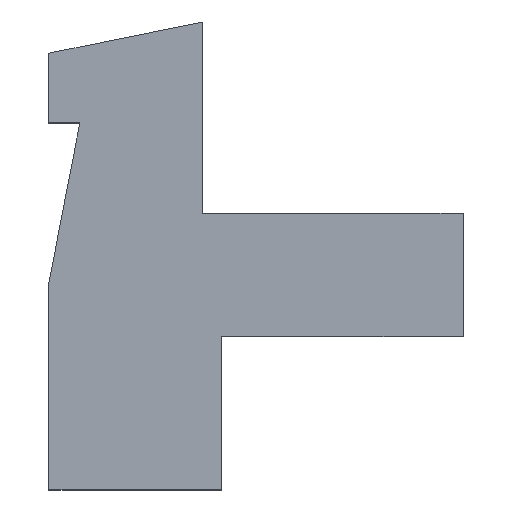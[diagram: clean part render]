
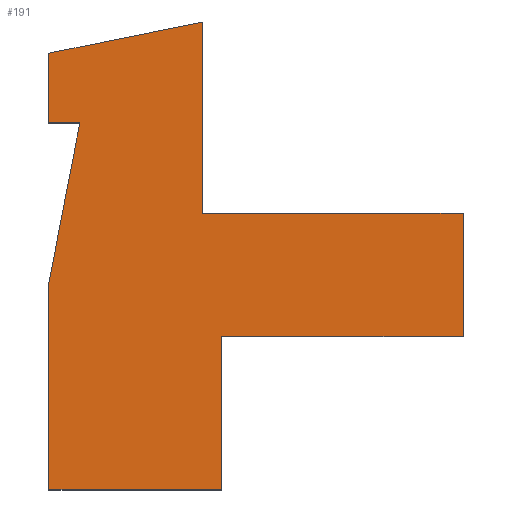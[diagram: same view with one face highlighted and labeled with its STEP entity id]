
A CAD part, top view. The second image highlights one B-rep face of the part: STEP entity #191.
In plain terms, the highlighted planar face has unit normal (0, 0, 1).
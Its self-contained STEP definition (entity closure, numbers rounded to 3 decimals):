
#6 = DIRECTION ( 'NONE',  ( 0., 1., 0. ) ) ;
#9 = VERTEX_POINT ( 'NONE', #388 ) ;
#41 = ORIENTED_EDGE ( 'NONE', *, *, #387, .F. ) ;
#51 = ORIENTED_EDGE ( 'NONE', *, *, #618, .T. ) ;
#52 = EDGE_CURVE ( 'NONE', #127, #202, #620, .T. ) ;
#57 = VERTEX_POINT ( 'NONE', #112 ) ;
#58 = EDGE_CURVE ( 'NONE', #484, #329, #366, .T. ) ;
#60 = CARTESIAN_POINT ( 'NONE',  ( -20.337, 1.836, 6. ) ) ;
#64 = LINE ( 'NONE', #419, #454 ) ;
#65 = ORIENTED_EDGE ( 'NONE', *, *, #556, .T. ) ;
#67 = EDGE_CURVE ( 'NONE', #299, #127, #131, .T. ) ;
#71 = DIRECTION ( 'NONE',  ( 0., 1., 0. ) ) ;
#77 = CARTESIAN_POINT ( 'NONE',  ( -24.719, 6.523, 6. ) ) ;
#83 = DIRECTION ( 'NONE',  ( 0., 0., 1. ) ) ;
#84 = CARTESIAN_POINT ( 'NONE',  ( -24.498, 7.643, 6. ) ) ;
#98 = VERTEX_POINT ( 'NONE', #396 ) ;
#102 = EDGE_CURVE ( 'NONE', #557, #202, #439, .T. ) ;
#104 = VECTOR ( 'NONE', #522, 1000. ) ;
#111 = VERTEX_POINT ( 'NONE', #302 ) ;
#112 = CARTESIAN_POINT ( 'NONE',  ( -24.326, 8.542, 6. ) ) ;
#117 = DIRECTION ( 'NONE',  ( 0., 1., 0. ) ) ;
#127 = VERTEX_POINT ( 'NONE', #595 ) ;
#131 = LINE ( 'NONE', #543, #187 ) ;
#146 = EDGE_LOOP ( 'NONE', ( #427, #240, #416, #489, #242, #367, #41, #269, #332, #65, #409, #51, #578, #223 ) ) ;
#148 = VECTOR ( 'NONE', #117, 1000. ) ;
#163 = CARTESIAN_POINT ( 'NONE',  ( -25.337, -8.414, 6. ) ) ;
#170 = LINE ( 'NONE', #575, #499 ) ;
#175 = DIRECTION ( 'NONE',  ( 1., 0., 0. ) ) ;
#186 = DIRECTION ( 'NONE',  ( -1., 0., 0. ) ) ;
#187 = VECTOR ( 'NONE', #450, 1000. ) ;
#191 = ADVANCED_FACE ( 'NONE', ( #399 ), #602, .T. ) ;
#193 = LINE ( 'NONE', #226, #104 ) ;
#202 = VERTEX_POINT ( 'NONE', #412 ) ;
#207 = CARTESIAN_POINT ( 'NONE',  ( -11.837, -8.414, 6. ) ) ;
#219 = DIRECTION ( 'NONE',  ( -1., 0., 0. ) ) ;
#223 = ORIENTED_EDGE ( 'NONE', *, *, #52, .F. ) ;
#225 = CARTESIAN_POINT ( 'NONE',  ( -11.837, 1.586, 6. ) ) ;
#226 = CARTESIAN_POINT ( 'NONE',  ( -19.7, -20.352, 6. ) ) ;
#228 = CARTESIAN_POINT ( 'NONE',  ( -25.337, 10.807, 6. ) ) ;
#229 = VECTOR ( 'NONE', #267, 1000. ) ;
#240 = ORIENTED_EDGE ( 'NONE', *, *, #241, .T. ) ;
#241 = EDGE_CURVE ( 'NONE', #299, #484, #193, .T. ) ;
#242 = ORIENTED_EDGE ( 'NONE', *, *, #394, .T. ) ;
#244 = VECTOR ( 'NONE', #311, 1000. ) ;
#257 = CARTESIAN_POINT ( 'NONE',  ( -19.7, 1.586, 6. ) ) ;
#265 = CARTESIAN_POINT ( 'NONE',  ( -24.498, 7.643, 6. ) ) ;
#267 = DIRECTION ( 'NONE',  ( -0.193, -0.981, 0. ) ) ;
#269 = ORIENTED_EDGE ( 'NONE', *, *, #485, .F. ) ;
#276 = VERTEX_POINT ( 'NONE', #228 ) ;
#299 = VERTEX_POINT ( 'NONE', #610 ) ;
#302 = CARTESIAN_POINT ( 'NONE',  ( -24.501, 7.643, 6. ) ) ;
#309 = CARTESIAN_POINT ( 'NONE',  ( -20.337, 11.825, 6. ) ) ;
#311 = DIRECTION ( 'NONE',  ( -0.191, -0.982, 0. ) ) ;
#312 = LINE ( 'NONE', #515, #483 ) ;
#313 = VECTOR ( 'NONE', #586, 1000. ) ;
#320 = EDGE_CURVE ( 'NONE', #9, #57, #64, .T. ) ;
#321 = VECTOR ( 'NONE', #524, 1000. ) ;
#326 = LINE ( 'NONE', #474, #321 ) ;
#329 = VERTEX_POINT ( 'NONE', #225 ) ;
#332 = ORIENTED_EDGE ( 'NONE', *, *, #320, .T. ) ;
#335 = EDGE_CURVE ( 'NONE', #111, #542, #312, .T. ) ;
#344 = AXIS2_PLACEMENT_3D ( 'NONE', #207, #83, #219 ) ;
#366 = LINE ( 'NONE', #436, #573 ) ;
#367 = ORIENTED_EDGE ( 'NONE', *, *, #531, .T. ) ;
#371 = LINE ( 'NONE', #555, #244 ) ;
#386 = CARTESIAN_POINT ( 'NONE',  ( -25.337, -8.414, 6. ) ) ;
#387 = EDGE_CURVE ( 'NONE', #276, #529, #326, .T. ) ;
#388 = CARTESIAN_POINT ( 'NONE',  ( -25.337, 8.542, 6. ) ) ;
#390 = CARTESIAN_POINT ( 'NONE',  ( -11.837, 5.586, 6. ) ) ;
#394 = EDGE_CURVE ( 'NONE', #492, #98, #170, .T. ) ;
#395 = CARTESIAN_POINT ( 'NONE',  ( -11.837, -8.414, 6. ) ) ;
#396 = CARTESIAN_POINT ( 'NONE',  ( -20.337, 5.586, 6. ) ) ;
#399 = FACE_OUTER_BOUND ( 'NONE', #146, .T. ) ;
#409 = ORIENTED_EDGE ( 'NONE', *, *, #335, .T. ) ;
#412 = CARTESIAN_POINT ( 'NONE',  ( -25.337, 3.339, 6. ) ) ;
#416 = ORIENTED_EDGE ( 'NONE', *, *, #58, .T. ) ;
#419 = CARTESIAN_POINT ( 'NONE',  ( -25.337, 8.542, 6. ) ) ;
#427 = ORIENTED_EDGE ( 'NONE', *, *, #67, .F. ) ;
#435 = EDGE_CURVE ( 'NONE', #329, #492, #554, .T. ) ;
#436 = CARTESIAN_POINT ( 'NONE',  ( -19.581, 1.586, 6. ) ) ;
#439 = LINE ( 'NONE', #495, #313 ) ;
#443 = LINE ( 'NONE', #163, #548 ) ;
#450 = DIRECTION ( 'NONE',  ( -1., 0., 0. ) ) ;
#454 = VECTOR ( 'NONE', #520, 1000. ) ;
#474 = CARTESIAN_POINT ( 'NONE',  ( -17.476, 12.407, 6. ) ) ;
#476 = VECTOR ( 'NONE', #6, 1000. ) ;
#483 = VECTOR ( 'NONE', #175, 1000. ) ;
#484 = VERTEX_POINT ( 'NONE', #257 ) ;
#485 = EDGE_CURVE ( 'NONE', #9, #276, #443, .T. ) ;
#489 = ORIENTED_EDGE ( 'NONE', *, *, #435, .T. ) ;
#492 = VERTEX_POINT ( 'NONE', #390 ) ;
#495 = CARTESIAN_POINT ( 'NONE',  ( -24.326, 8.542, 6. ) ) ;
#496 = DIRECTION ( 'NONE',  ( 0., 1., 0. ) ) ;
#497 = LINE ( 'NONE', #60, #148 ) ;
#499 = VECTOR ( 'NONE', #186, 1000. ) ;
#515 = CARTESIAN_POINT ( 'NONE',  ( -28.016, 7.643, 6. ) ) ;
#520 = DIRECTION ( 'NONE',  ( 1., 0., 0. ) ) ;
#522 = DIRECTION ( 'NONE',  ( 0., 1., 0. ) ) ;
#524 = DIRECTION ( 'NONE',  ( 0.98, 0.199, 0. ) ) ;
#529 = VERTEX_POINT ( 'NONE', #309 ) ;
#531 = EDGE_CURVE ( 'NONE', #98, #529, #497, .T. ) ;
#538 = VECTOR ( 'NONE', #71, 1000. ) ;
#539 = DIRECTION ( 'NONE',  ( 1., 0., 0. ) ) ;
#542 = VERTEX_POINT ( 'NONE', #265 ) ;
#543 = CARTESIAN_POINT ( 'NONE',  ( -18.587, -3.414, 6. ) ) ;
#546 = LINE ( 'NONE', #84, #229 ) ;
#548 = VECTOR ( 'NONE', #496, 1000. ) ;
#554 = LINE ( 'NONE', #395, #538 ) ;
#555 = CARTESIAN_POINT ( 'NONE',  ( -24.326, 8.542, 6. ) ) ;
#556 = EDGE_CURVE ( 'NONE', #57, #111, #371, .T. ) ;
#557 = VERTEX_POINT ( 'NONE', #77 ) ;
#573 = VECTOR ( 'NONE', #539, 1000. ) ;
#575 = CARTESIAN_POINT ( 'NONE',  ( -16.087, 5.586, 6. ) ) ;
#578 = ORIENTED_EDGE ( 'NONE', *, *, #102, .T. ) ;
#586 = DIRECTION ( 'NONE',  ( -0.191, -0.982, 0. ) ) ;
#595 = CARTESIAN_POINT ( 'NONE',  ( -25.337, -3.414, 6. ) ) ;
#602 = PLANE ( 'NONE',  #344 ) ;
#610 = CARTESIAN_POINT ( 'NONE',  ( -19.7, -3.414, 6. ) ) ;
#618 = EDGE_CURVE ( 'NONE', #542, #557, #546, .T. ) ;
#620 = LINE ( 'NONE', #386, #476 ) ;
